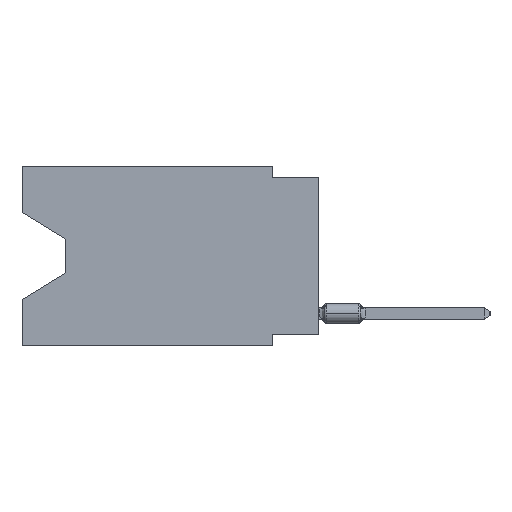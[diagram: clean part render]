
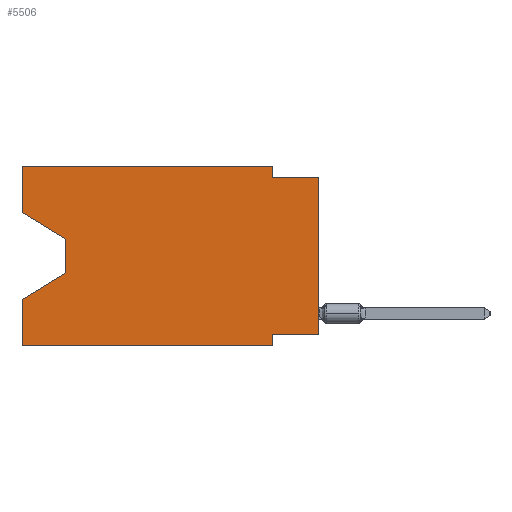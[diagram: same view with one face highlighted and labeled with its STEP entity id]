
A CAD part, left-side view. The second image highlights one B-rep face of the part: STEP entity #5506.
In plain terms, the highlighted planar face has unit normal (-1, 0, 0).
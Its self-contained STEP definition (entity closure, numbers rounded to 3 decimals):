
#330 = LINE ( 'NONE', #35659, #354 ) ;
#354 = VECTOR ( 'NONE', #4016, 1000. ) ;
#993 = LINE ( 'NONE', #32187, #6182 ) ;
#1031 = VECTOR ( 'NONE', #24672, 1000. ) ;
#1260 = DIRECTION ( 'NONE',  ( 0., 0., -1. ) ) ;
#1310 = VECTOR ( 'NONE', #19670, 1000. ) ;
#1332 = EDGE_CURVE ( 'NONE', #26647, #14286, #993, .T. ) ;
#1594 = DIRECTION ( 'NONE',  ( 1., 0., 0. ) ) ;
#1960 = EDGE_CURVE ( 'NONE', #23886, #21692, #20390, .T. ) ;
#2356 = EDGE_CURVE ( 'NONE', #12840, #21692, #33919, .T. ) ;
#3754 = VERTEX_POINT ( 'NONE', #42868 ) ;
#4016 = DIRECTION ( 'NONE',  ( 0., 0., -1. ) ) ;
#5506 = ADVANCED_FACE ( 'NONE', ( #29550 ), #25866, .F. ) ;
#5546 = VECTOR ( 'NONE', #36446, 1000. ) ;
#5950 = VECTOR ( 'NONE', #39381, 1000. ) ;
#6030 = ORIENTED_EDGE ( 'NONE', *, *, #7947, .F. ) ;
#6182 = VECTOR ( 'NONE', #18082, 1000. ) ;
#6685 = ORIENTED_EDGE ( 'NONE', *, *, #9942, .F. ) ;
#7676 = LINE ( 'NONE', #25903, #31640 ) ;
#7947 = EDGE_CURVE ( 'NONE', #26647, #20315, #7676, .T. ) ;
#8969 = CARTESIAN_POINT ( 'NONE',  ( 0., 13.97, -5.893 ) ) ;
#9867 = CARTESIAN_POINT ( 'NONE',  ( 0., 0., -9.271 ) ) ;
#9942 = EDGE_CURVE ( 'NONE', #45205, #20195, #41535, .T. ) ;
#10277 = EDGE_CURVE ( 'NONE', #40648, #12266, #16672, .T. ) ;
#10668 = ORIENTED_EDGE ( 'NONE', *, *, #10277, .F. ) ;
#11578 = DIRECTION ( 'NONE',  ( 0., 0., 1. ) ) ;
#11613 = ORIENTED_EDGE ( 'NONE', *, *, #1332, .T. ) ;
#11761 = CARTESIAN_POINT ( 'NONE',  ( 0., 0., 0. ) ) ;
#12266 = VERTEX_POINT ( 'NONE', #15060 ) ;
#12503 = LINE ( 'NONE', #16420, #1310 ) ;
#12529 = LINE ( 'NONE', #26629, #12982 ) ;
#12840 = VERTEX_POINT ( 'NONE', #13985 ) ;
#12982 = VECTOR ( 'NONE', #1260, 1000. ) ;
#13985 = CARTESIAN_POINT ( 'NONE',  ( 0., 13.97, -5.893 ) ) ;
#14286 = VERTEX_POINT ( 'NONE', #44900 ) ;
#14440 = CARTESIAN_POINT ( 'NONE',  ( 0., 16.383, 0. ) ) ;
#14526 = AXIS2_PLACEMENT_3D ( 'NONE', #40186, #1594, #26303 ) ;
#14798 = ORIENTED_EDGE ( 'NONE', *, *, #26793, .T. ) ;
#15060 = CARTESIAN_POINT ( 'NONE',  ( 0., 2.54, -0.635 ) ) ;
#16140 = CARTESIAN_POINT ( 'NONE',  ( 0., 0., -9.271 ) ) ;
#16420 = CARTESIAN_POINT ( 'NONE',  ( 0., 16.383, -9.906 ) ) ;
#16672 = LINE ( 'NONE', #38192, #22204 ) ;
#16919 = DIRECTION ( 'NONE',  ( 0., 0., 1. ) ) ;
#18082 = DIRECTION ( 'NONE',  ( 0., -0.855, -0.519 ) ) ;
#18875 = LINE ( 'NONE', #22356, #5546 ) ;
#19670 = DIRECTION ( 'NONE',  ( 0., -1., 0. ) ) ;
#20195 = VERTEX_POINT ( 'NONE', #27852 ) ;
#20315 = VERTEX_POINT ( 'NONE', #14440 ) ;
#20390 = LINE ( 'NONE', #23632, #24696 ) ;
#21064 = DIRECTION ( 'NONE',  ( 0., 0., -1. ) ) ;
#21692 = VERTEX_POINT ( 'NONE', #28625 ) ;
#22094 = VECTOR ( 'NONE', #36263, 1000. ) ;
#22204 = VECTOR ( 'NONE', #21064, 1000. ) ;
#22356 = CARTESIAN_POINT ( 'NONE',  ( 0., 16.383, 0. ) ) ;
#22473 = VECTOR ( 'NONE', #30679, 1000. ) ;
#23632 = CARTESIAN_POINT ( 'NONE',  ( 0., 16.383, 0. ) ) ;
#23886 = VERTEX_POINT ( 'NONE', #37492 ) ;
#24672 = DIRECTION ( 'NONE',  ( 0., -1., 0. ) ) ;
#24696 = VECTOR ( 'NONE', #16919, 1000. ) ;
#25713 = ORIENTED_EDGE ( 'NONE', *, *, #38243, .T. ) ;
#25866 = PLANE ( 'NONE',  #14526 ) ;
#25903 = CARTESIAN_POINT ( 'NONE',  ( 0., 16.383, 0. ) ) ;
#26303 = DIRECTION ( 'NONE',  ( 0., 0., -1. ) ) ;
#26629 = CARTESIAN_POINT ( 'NONE',  ( 0., 13.97, -4.013 ) ) ;
#26647 = VERTEX_POINT ( 'NONE', #39620 ) ;
#26793 = EDGE_CURVE ( 'NONE', #14286, #12840, #12529, .T. ) ;
#26825 = ORIENTED_EDGE ( 'NONE', *, *, #28630, .T. ) ;
#27852 = CARTESIAN_POINT ( 'NONE',  ( 0., 2.54, -9.271 ) ) ;
#28625 = CARTESIAN_POINT ( 'NONE',  ( 0., 16.383, -7.36 ) ) ;
#28630 = EDGE_CURVE ( 'NONE', #45205, #3754, #39294, .T. ) ;
#29550 = FACE_OUTER_BOUND ( 'NONE', #40937, .T. ) ;
#30484 = CARTESIAN_POINT ( 'NONE',  ( 0., 2.54, 0. ) ) ;
#30679 = DIRECTION ( 'NONE',  ( 0., 0.855, -0.519 ) ) ;
#31640 = VECTOR ( 'NONE', #11578, 1000. ) ;
#31920 = ORIENTED_EDGE ( 'NONE', *, *, #1960, .F. ) ;
#32187 = CARTESIAN_POINT ( 'NONE',  ( 0., 16.383, -2.546 ) ) ;
#33608 = EDGE_CURVE ( 'NONE', #12266, #3754, #38544, .T. ) ;
#33919 = LINE ( 'NONE', #8969, #22473 ) ;
#35659 = CARTESIAN_POINT ( 'NONE',  ( 0., 2.54, -9.906 ) ) ;
#36263 = DIRECTION ( 'NONE',  ( 0., 0., 1. ) ) ;
#36446 = DIRECTION ( 'NONE',  ( 0., -1., 0. ) ) ;
#36734 = ORIENTED_EDGE ( 'NONE', *, *, #45523, .F. ) ;
#37333 = CARTESIAN_POINT ( 'NONE',  ( 0., 2.54, -9.906 ) ) ;
#37492 = CARTESIAN_POINT ( 'NONE',  ( 0., 16.383, -9.906 ) ) ;
#38192 = CARTESIAN_POINT ( 'NONE',  ( 0., 2.54, 0. ) ) ;
#38243 = EDGE_CURVE ( 'NONE', #23886, #42908, #12503, .T. ) ;
#38544 = LINE ( 'NONE', #42236, #1031 ) ;
#39294 = LINE ( 'NONE', #11761, #22094 ) ;
#39381 = DIRECTION ( 'NONE',  ( 0., 1., 0. ) ) ;
#39620 = CARTESIAN_POINT ( 'NONE',  ( 0., 16.383, -2.546 ) ) ;
#39803 = ORIENTED_EDGE ( 'NONE', *, *, #2356, .T. ) ;
#40186 = CARTESIAN_POINT ( 'NONE',  ( 0., 16.383, 0. ) ) ;
#40648 = VERTEX_POINT ( 'NONE', #30484 ) ;
#40937 = EDGE_LOOP ( 'NONE', ( #11613, #14798, #39803, #31920, #25713, #44821, #6685, #26825, #43920, #10668, #36734, #6030 ) ) ;
#41535 = LINE ( 'NONE', #9867, #5950 ) ;
#42236 = CARTESIAN_POINT ( 'NONE',  ( 0., 0., -0.635 ) ) ;
#42868 = CARTESIAN_POINT ( 'NONE',  ( 0., 0., -0.635 ) ) ;
#42908 = VERTEX_POINT ( 'NONE', #37333 ) ;
#43920 = ORIENTED_EDGE ( 'NONE', *, *, #33608, .F. ) ;
#44437 = EDGE_CURVE ( 'NONE', #20195, #42908, #330, .T. ) ;
#44821 = ORIENTED_EDGE ( 'NONE', *, *, #44437, .F. ) ;
#44900 = CARTESIAN_POINT ( 'NONE',  ( 0., 13.97, -4.013 ) ) ;
#45205 = VERTEX_POINT ( 'NONE', #16140 ) ;
#45523 = EDGE_CURVE ( 'NONE', #20315, #40648, #18875, .T. ) ;
